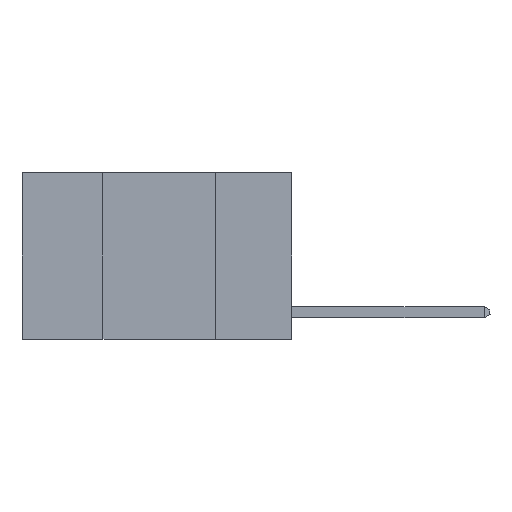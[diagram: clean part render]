
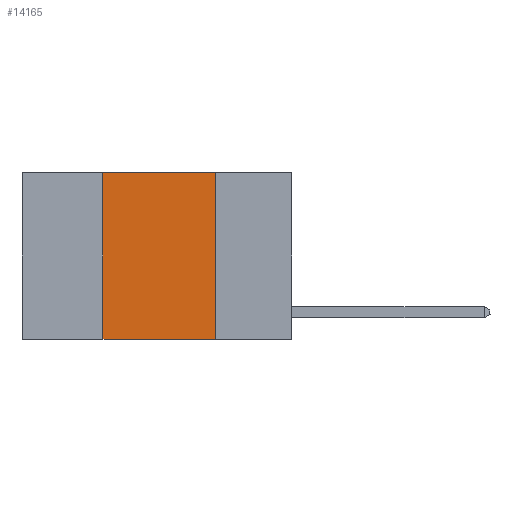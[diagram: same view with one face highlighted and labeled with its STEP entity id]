
A CAD part, left-side view. The second image highlights one B-rep face of the part: STEP entity #14165.
In plain terms, the highlighted planar face has unit normal (-1, 0, 0).
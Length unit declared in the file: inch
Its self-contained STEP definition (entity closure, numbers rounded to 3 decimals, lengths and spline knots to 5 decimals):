
#631 = CARTESIAN_POINT ( 'NONE',  ( 0., 0.6, 0. ) ) ;
#704 = DIRECTION ( 'NONE',  ( 0., 0., -1. ) ) ;
#831 = AXIS2_PLACEMENT_3D ( 'NONE', #631, #10613, #704 ) ;
#889 = DIRECTION ( 'NONE',  ( 0., 0., -1. ) ) ;
#1954 = CARTESIAN_POINT ( 'NONE',  ( 0., 0.6, 0. ) ) ;
#2795 = ORIENTED_EDGE ( 'NONE', *, *, #15294, .F. ) ;
#2903 = CARTESIAN_POINT ( 'NONE',  ( 0., 0.6, -0.37 ) ) ;
#4328 = CARTESIAN_POINT ( 'NONE',  ( 0., 0.17, -0.37 ) ) ;
#4568 = DIRECTION ( 'NONE',  ( 0., -1., 0. ) ) ;
#4948 = VECTOR ( 'NONE', #7024, 39.37008 ) ;
#5467 = LINE ( 'NONE', #1954, #4948 ) ;
#6308 = CARTESIAN_POINT ( 'NONE',  ( 0., 0.42, 0. ) ) ;
#6393 = VERTEX_POINT ( 'NONE', #10389 ) ;
#6466 = ORIENTED_EDGE ( 'NONE', *, *, #13168, .F. ) ;
#6827 = EDGE_LOOP ( 'NONE', ( #2795, #9610, #6466, #11057 ) ) ;
#6982 = CARTESIAN_POINT ( 'NONE',  ( 0., 0.42, 0. ) ) ;
#7024 = DIRECTION ( 'NONE',  ( 0., -1., 0. ) ) ;
#7803 = VECTOR ( 'NONE', #4568, 39.37008 ) ;
#7856 = LINE ( 'NONE', #12440, #20720 ) ;
#7962 = DIRECTION ( 'NONE',  ( 0., 0., 1. ) ) ;
#8347 = LINE ( 'NONE', #2903, #7803 ) ;
#8748 = LINE ( 'NONE', #6308, #20568 ) ;
#9610 = ORIENTED_EDGE ( 'NONE', *, *, #18008, .F. ) ;
#9880 = EDGE_CURVE ( 'NONE', #6393, #10482, #8347, .T. ) ;
#10389 = CARTESIAN_POINT ( 'NONE',  ( 0., 0.42, -0.37 ) ) ;
#10482 = VERTEX_POINT ( 'NONE', #4328 ) ;
#10613 = DIRECTION ( 'NONE',  ( 1., 0., 0. ) ) ;
#11057 = ORIENTED_EDGE ( 'NONE', *, *, #9880, .T. ) ;
#12045 = FACE_OUTER_BOUND ( 'NONE', #6827, .T. ) ;
#12440 = CARTESIAN_POINT ( 'NONE',  ( 0., 0.17, 0. ) ) ;
#13168 = EDGE_CURVE ( 'NONE', #6393, #16863, #8748, .T. ) ;
#14165 = ADVANCED_FACE ( 'NONE', ( #12045 ), #20205, .F. ) ;
#15294 = EDGE_CURVE ( 'NONE', #18882, #10482, #7856, .T. ) ;
#16863 = VERTEX_POINT ( 'NONE', #6982 ) ;
#17685 = CARTESIAN_POINT ( 'NONE',  ( 0., 0.17, 0. ) ) ;
#18008 = EDGE_CURVE ( 'NONE', #16863, #18882, #5467, .T. ) ;
#18882 = VERTEX_POINT ( 'NONE', #17685 ) ;
#20205 = PLANE ( 'NONE',  #831 ) ;
#20568 = VECTOR ( 'NONE', #7962, 39.37008 ) ;
#20720 = VECTOR ( 'NONE', #889, 39.37008 ) ;
